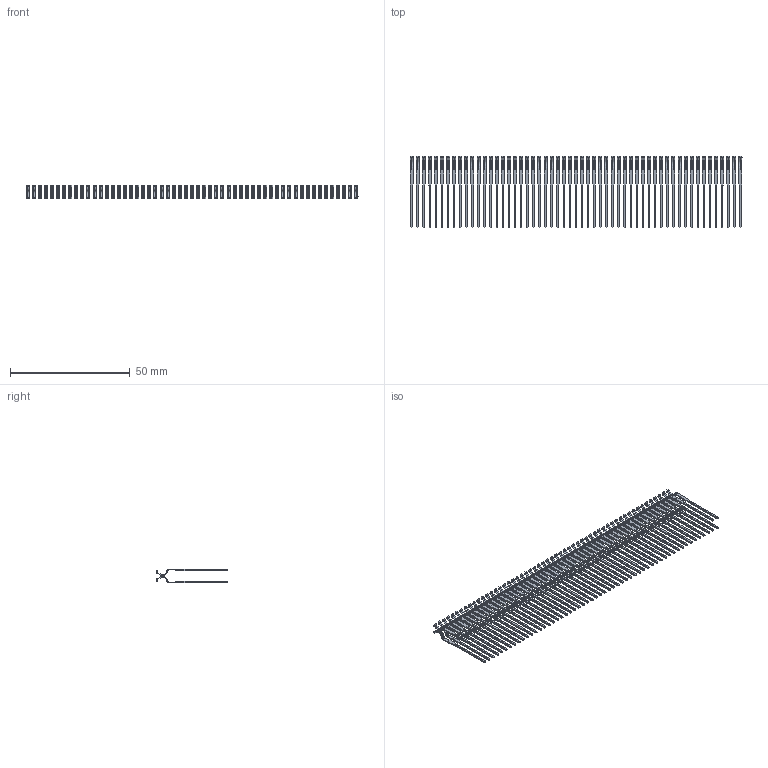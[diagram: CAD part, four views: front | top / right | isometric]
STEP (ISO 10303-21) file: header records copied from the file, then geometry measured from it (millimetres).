
FILE_DESCRIPTION (( 'STEP AP203' ), '1' );
FILE_NAME ('395-110-542-212.STEP', '2019-10-27T11:07:34', ( '' ), ( '' ), 'SwSTEP 2.0', 'SolidWorks 2016', '' );
FILE_SCHEMA (( 'CONFIG_CONTROL_DESIGN' ));
Length unit declared in the file: inch
Products named in the file (3): 345 Part_Flush Mounting Lugs - Side Mount; 345-292-001_345-293-142; 395-110-542-212
Assembly tree (111 placements, depth 2):
  395-110-542-212
    345 Part_Flush Mounting Lugs - Side Mount
    345-292-001_345-293-142  x110
Bounding box: 138.43 x 29.72 x 5.71 mm (x, y, z)
Volume: 1504.3 mm3; surface area: 10236 mm2
Topology: 110 solids, 110 shells, 4620 faces, 13420 edges, 8800 vertices
Faces by surface type: plane 2860, cylinder 1760
Entity records: 41425 total; most frequent: CARTESIAN_POINT 6932, ORIENTED_EDGE 6866, DIRECTION 6097, EDGE_CURVE 3433, VECTOR 3081, LINE 3081, VERTEX_POINT 2286, AXIS2_PLACEMENT_3D 1508
